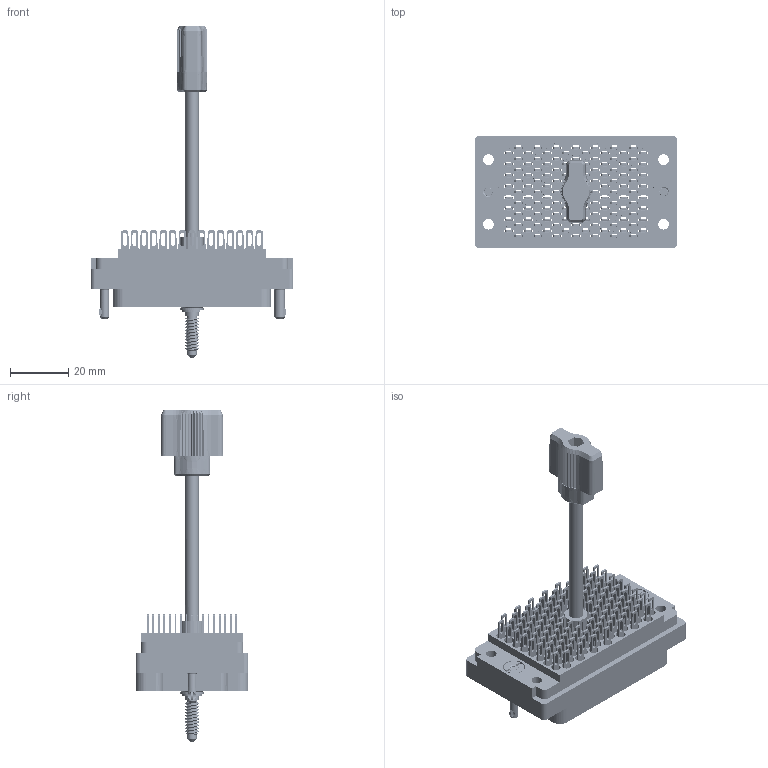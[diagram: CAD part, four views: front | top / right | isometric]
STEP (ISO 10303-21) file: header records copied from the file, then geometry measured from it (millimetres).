
FILE_DESCRIPTION (( 'STEP AP203' ), '1' );
FILE_NAME ('516-120-500-301.STEP', '2020-03-11T02:29:53', ( '' ), ( '' ), 'SwSTEP 2.0', 'SolidWorks 2016', '' );
FILE_SCHEMA (( 'CONFIG_CONTROL_DESIGN' ));
Length unit declared in the file: inch
Products named in the file (13): Actuating Screw Assy 090-120; 516-250-091-111; 516-252-091-102; Grub Screw; 516 Plug Insulator_120; 516-253-095-100; 516-251-095-100; 516-222-090-102_091; 516-253-190-107; 516-292-001_500 Contact; 516-222-090-102_090; 516-120-500-301; 516-254-091-109
Assembly tree (133 placements, depth 3):
  516-120-500-301
    516 Plug Insulator_120
    516-292-001_500 Contact  x120
    516-252-091-102  x2
    516-222-090-102_090
    Actuating Screw Assy 090-120
      516-251-095-100
      516-254-091-109
      516-253-095-100  x2
      516-253-190-107
      516-250-091-111
      Grub Screw
    516-222-090-102_091
Bounding box: 69.85 x 38.73 x 114.34 mm (x, y, z)
Volume: 29393.7 mm3; surface area: 54059.3 mm2
Topology: 132 solids, 132 shells, 11975 faces, 34689 edges, 23002 vertices
Faces by surface type: plane 7115, cylinder 3993, bspline 767, cone 96, torus 4
Entity records: 113535 total; most frequent: CARTESIAN_POINT 30444, ORIENTED_EDGE 16838, DIRECTION 16023, EDGE_CURVE 8419, VECTOR 6009, LINE 6009, VERTEX_POINT 5568, AXIS2_PLACEMENT_3D 5007
